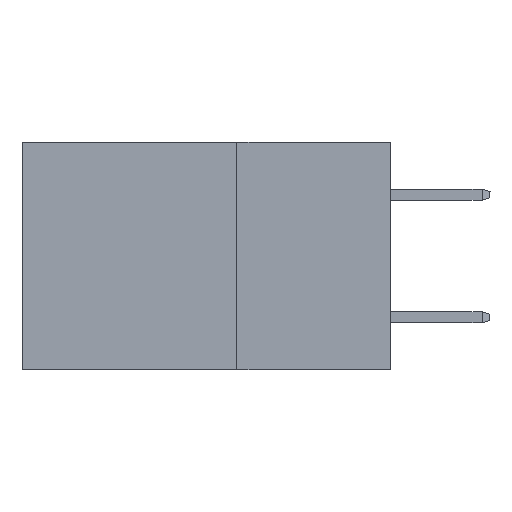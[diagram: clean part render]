
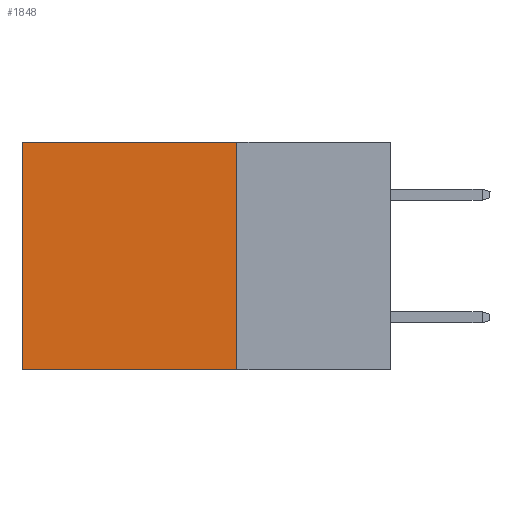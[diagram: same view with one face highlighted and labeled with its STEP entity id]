
A CAD part, left-side view. The second image highlights one B-rep face of the part: STEP entity #1848.
In plain terms, the highlighted planar face has unit normal (-1, 0, 0).
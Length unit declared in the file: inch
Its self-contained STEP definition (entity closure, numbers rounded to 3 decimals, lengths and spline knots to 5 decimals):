
#1034 = EDGE_CURVE ( 'NONE', #6290, #2529, #11428, .T. ) ;
#1289 = DIRECTION ( 'NONE',  ( 0., 0., -1. ) ) ;
#1349 = VECTOR ( 'NONE', #1289, 39.37008 ) ;
#1848 = ADVANCED_FACE ( 'NONE', ( #2904 ), #9596, .F. ) ;
#2099 = LINE ( 'NONE', #13408, #6165 ) ;
#2365 = CARTESIAN_POINT ( 'NONE',  ( 0.2875, 0.25, 0. ) ) ;
#2529 = VERTEX_POINT ( 'NONE', #3499 ) ;
#2904 = FACE_OUTER_BOUND ( 'NONE', #3687, .T. ) ;
#3053 = AXIS2_PLACEMENT_3D ( 'NONE', #6634, #12418, #15198 ) ;
#3499 = CARTESIAN_POINT ( 'NONE',  ( 0.2875, 0.25, -0.37 ) ) ;
#3687 = EDGE_LOOP ( 'NONE', ( #4147, #7656, #10911, #9184 ) ) ;
#3813 = LINE ( 'NONE', #2365, #11841 ) ;
#3846 = CARTESIAN_POINT ( 'NONE',  ( 0.2875, 0.25, 0. ) ) ;
#4147 = ORIENTED_EDGE ( 'NONE', *, *, #10429, .T. ) ;
#4776 = VECTOR ( 'NONE', #7279, 39.37008 ) ;
#4853 = EDGE_CURVE ( 'NONE', #2529, #7425, #2099, .T. ) ;
#5179 = CARTESIAN_POINT ( 'NONE',  ( 0.2875, 0.6, 0. ) ) ;
#6165 = VECTOR ( 'NONE', #6445, 39.37008 ) ;
#6290 = VERTEX_POINT ( 'NONE', #3846 ) ;
#6445 = DIRECTION ( 'NONE',  ( 0., 1., 0. ) ) ;
#6634 = CARTESIAN_POINT ( 'NONE',  ( 0.2875, 0.25, 0. ) ) ;
#6648 = VERTEX_POINT ( 'NONE', #10086 ) ;
#7185 = CARTESIAN_POINT ( 'NONE',  ( 0.2875, 0.25, 0. ) ) ;
#7279 = DIRECTION ( 'NONE',  ( 0., 0., -1. ) ) ;
#7425 = VERTEX_POINT ( 'NONE', #13486 ) ;
#7656 = ORIENTED_EDGE ( 'NONE', *, *, #4853, .F. ) ;
#9184 = ORIENTED_EDGE ( 'NONE', *, *, #14333, .T. ) ;
#9254 = LINE ( 'NONE', #5179, #1349 ) ;
#9596 = PLANE ( 'NONE',  #3053 ) ;
#10086 = CARTESIAN_POINT ( 'NONE',  ( 0.2875, 0.6, 0. ) ) ;
#10429 = EDGE_CURVE ( 'NONE', #6648, #7425, #9254, .T. ) ;
#10794 = DIRECTION ( 'NONE',  ( 0., 1., 0. ) ) ;
#10911 = ORIENTED_EDGE ( 'NONE', *, *, #1034, .F. ) ;
#11428 = LINE ( 'NONE', #7185, #4776 ) ;
#11841 = VECTOR ( 'NONE', #10794, 39.37008 ) ;
#12418 = DIRECTION ( 'NONE',  ( 1., 0., 0. ) ) ;
#13408 = CARTESIAN_POINT ( 'NONE',  ( 0.2875, 0.25, -0.37 ) ) ;
#13486 = CARTESIAN_POINT ( 'NONE',  ( 0.2875, 0.6, -0.37 ) ) ;
#14333 = EDGE_CURVE ( 'NONE', #6290, #6648, #3813, .T. ) ;
#15198 = DIRECTION ( 'NONE',  ( 0., 0., -1. ) ) ;
